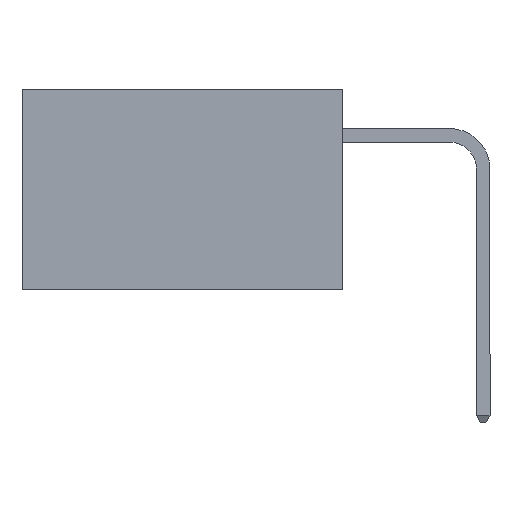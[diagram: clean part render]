
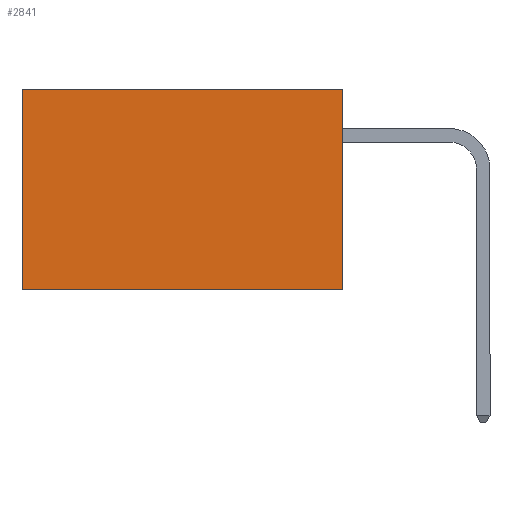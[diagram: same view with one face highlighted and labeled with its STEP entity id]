
A CAD part, left-side view. The second image highlights one B-rep face of the part: STEP entity #2841.
In plain terms, the highlighted planar face has unit normal (-1, 0, 0).
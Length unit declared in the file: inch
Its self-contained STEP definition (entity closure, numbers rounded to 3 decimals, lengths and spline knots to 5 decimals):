
#729 = EDGE_CURVE ( 'NONE', #5988, #2550, #4123, .T. ) ;
#1264 = CARTESIAN_POINT ( 'NONE',  ( 0.277, 0., -0.37 ) ) ;
#1827 = VERTEX_POINT ( 'NONE', #3745 ) ;
#2517 = LINE ( 'NONE', #6670, #6059 ) ;
#2550 = VERTEX_POINT ( 'NONE', #7787 ) ;
#2574 = EDGE_CURVE ( 'NONE', #2550, #7405, #2517, .T. ) ;
#2820 = ORIENTED_EDGE ( 'NONE', *, *, #3156, .T. ) ;
#2841 = ADVANCED_FACE ( 'NONE', ( #5940 ), #4159, .F. ) ;
#2900 = ORIENTED_EDGE ( 'NONE', *, *, #2574, .F. ) ;
#3156 = EDGE_CURVE ( 'NONE', #1827, #7405, #5827, .T. ) ;
#3745 = CARTESIAN_POINT ( 'NONE',  ( 0.277, 0.59, 0. ) ) ;
#3855 = DIRECTION ( 'NONE',  ( 0., 0., -1. ) ) ;
#3998 = DIRECTION ( 'NONE',  ( 0., 0., -1. ) ) ;
#4123 = LINE ( 'NONE', #8094, #5763 ) ;
#4159 = PLANE ( 'NONE',  #7657 ) ;
#4377 = DIRECTION ( 'NONE',  ( 0., 1., 0. ) ) ;
#4453 = VECTOR ( 'NONE', #4377, 39.37008 ) ;
#5466 = CARTESIAN_POINT ( 'NONE',  ( 0.277, 0., 0. ) ) ;
#5763 = VECTOR ( 'NONE', #7027, 39.37008 ) ;
#5827 = LINE ( 'NONE', #8732, #8760 ) ;
#5940 = FACE_OUTER_BOUND ( 'NONE', #8315, .T. ) ;
#5988 = VERTEX_POINT ( 'NONE', #6857 ) ;
#6059 = VECTOR ( 'NONE', #7317, 39.37008 ) ;
#6277 = LINE ( 'NONE', #5466, #4453 ) ;
#6479 = EDGE_CURVE ( 'NONE', #5988, #1827, #6277, .T. ) ;
#6670 = CARTESIAN_POINT ( 'NONE',  ( 0.277, 0., -0.37 ) ) ;
#6857 = CARTESIAN_POINT ( 'NONE',  ( 0.277, 0., 0. ) ) ;
#7027 = DIRECTION ( 'NONE',  ( 0., 0., -1. ) ) ;
#7317 = DIRECTION ( 'NONE',  ( 0., 1., 0. ) ) ;
#7405 = VERTEX_POINT ( 'NONE', #7911 ) ;
#7657 = AXIS2_PLACEMENT_3D ( 'NONE', #1264, #8736, #3998 ) ;
#7787 = CARTESIAN_POINT ( 'NONE',  ( 0.277, 0., -0.37 ) ) ;
#7911 = CARTESIAN_POINT ( 'NONE',  ( 0.277, 0.59, -0.37 ) ) ;
#8094 = CARTESIAN_POINT ( 'NONE',  ( 0.277, 0., -0.37 ) ) ;
#8110 = ORIENTED_EDGE ( 'NONE', *, *, #729, .F. ) ;
#8168 = ORIENTED_EDGE ( 'NONE', *, *, #6479, .T. ) ;
#8315 = EDGE_LOOP ( 'NONE', ( #2820, #2900, #8110, #8168 ) ) ;
#8732 = CARTESIAN_POINT ( 'NONE',  ( 0.277, 0.59, -0.37 ) ) ;
#8736 = DIRECTION ( 'NONE',  ( 1., 0., 0. ) ) ;
#8760 = VECTOR ( 'NONE', #3855, 39.37008 ) ;
